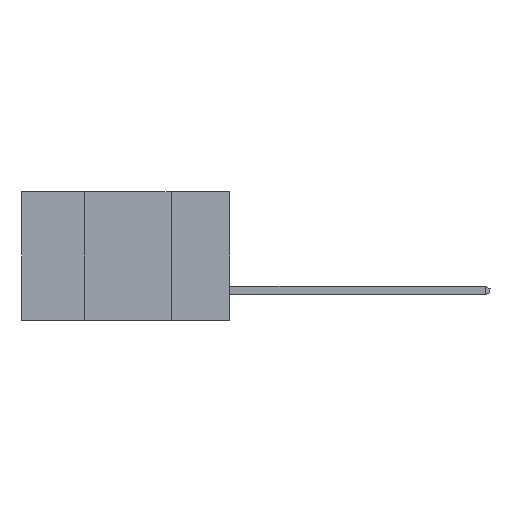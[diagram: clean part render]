
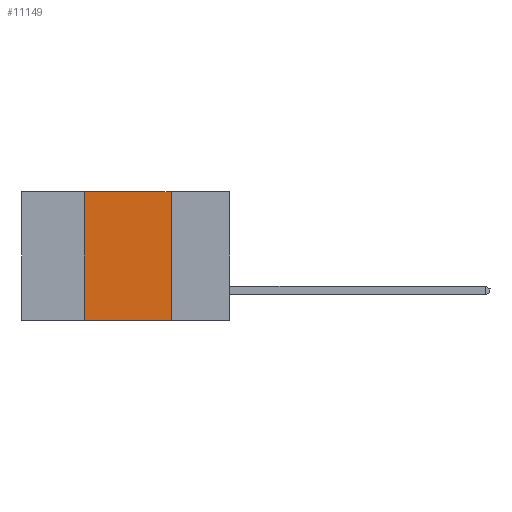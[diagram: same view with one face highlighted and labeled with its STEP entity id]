
A CAD part, left-side view. The second image highlights one B-rep face of the part: STEP entity #11149.
In plain terms, the highlighted planar face has unit normal (-1, 0, 0).
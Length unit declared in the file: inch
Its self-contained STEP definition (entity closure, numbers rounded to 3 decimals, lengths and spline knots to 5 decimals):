
#453 = LINE ( 'NONE', #4510, #7638 ) ;
#649 = CARTESIAN_POINT ( 'NONE',  ( 0., 0.6, -0.37 ) ) ;
#862 = LINE ( 'NONE', #3896, #9520 ) ;
#1117 = VECTOR ( 'NONE', #1771, 39.37008 ) ;
#1473 = DIRECTION ( 'NONE',  ( 0., 0., -1. ) ) ;
#1723 = CARTESIAN_POINT ( 'NONE',  ( 0., 0.17, 0. ) ) ;
#1771 = DIRECTION ( 'NONE',  ( 0., 0., 1. ) ) ;
#2003 = EDGE_CURVE ( 'NONE', #6702, #11780, #6639, .T. ) ;
#2922 = VECTOR ( 'NONE', #10664, 39.37008 ) ;
#3034 = DIRECTION ( 'NONE',  ( 0., 0., -1. ) ) ;
#3722 = CARTESIAN_POINT ( 'NONE',  ( 0., 0.42, -0.37 ) ) ;
#3830 = EDGE_CURVE ( 'NONE', #11780, #7041, #862, .T. ) ;
#3896 = CARTESIAN_POINT ( 'NONE',  ( 0., 0.6, 0. ) ) ;
#4341 = ORIENTED_EDGE ( 'NONE', *, *, #2003, .F. ) ;
#4510 = CARTESIAN_POINT ( 'NONE',  ( 0., 0.17, -0.37 ) ) ;
#4784 = DIRECTION ( 'NONE',  ( 0., -1., 0. ) ) ;
#6546 = AXIS2_PLACEMENT_3D ( 'NONE', #12556, #6737, #3034 ) ;
#6639 = LINE ( 'NONE', #3722, #1117 ) ;
#6702 = VERTEX_POINT ( 'NONE', #6964 ) ;
#6737 = DIRECTION ( 'NONE',  ( 1., 0., 0. ) ) ;
#6964 = CARTESIAN_POINT ( 'NONE',  ( 0., 0.42, -0.37 ) ) ;
#7041 = VERTEX_POINT ( 'NONE', #1723 ) ;
#7638 = VECTOR ( 'NONE', #1473, 39.37008 ) ;
#7749 = FACE_OUTER_BOUND ( 'NONE', #8128, .T. ) ;
#7851 = ORIENTED_EDGE ( 'NONE', *, *, #11911, .F. ) ;
#7982 = CARTESIAN_POINT ( 'NONE',  ( 0., 0.42, 0. ) ) ;
#8128 = EDGE_LOOP ( 'NONE', ( #7851, #9721, #4341, #11133 ) ) ;
#8955 = VERTEX_POINT ( 'NONE', #11742 ) ;
#9520 = VECTOR ( 'NONE', #4784, 39.37008 ) ;
#9614 = PLANE ( 'NONE',  #6546 ) ;
#9721 = ORIENTED_EDGE ( 'NONE', *, *, #3830, .F. ) ;
#9915 = EDGE_CURVE ( 'NONE', #6702, #8955, #11402, .T. ) ;
#10664 = DIRECTION ( 'NONE',  ( 0., -1., 0. ) ) ;
#11133 = ORIENTED_EDGE ( 'NONE', *, *, #9915, .T. ) ;
#11149 = ADVANCED_FACE ( 'NONE', ( #7749 ), #9614, .F. ) ;
#11402 = LINE ( 'NONE', #649, #2922 ) ;
#11742 = CARTESIAN_POINT ( 'NONE',  ( 0., 0.17, -0.37 ) ) ;
#11780 = VERTEX_POINT ( 'NONE', #7982 ) ;
#11911 = EDGE_CURVE ( 'NONE', #7041, #8955, #453, .T. ) ;
#12556 = CARTESIAN_POINT ( 'NONE',  ( 0., 0.6, 0. ) ) ;
